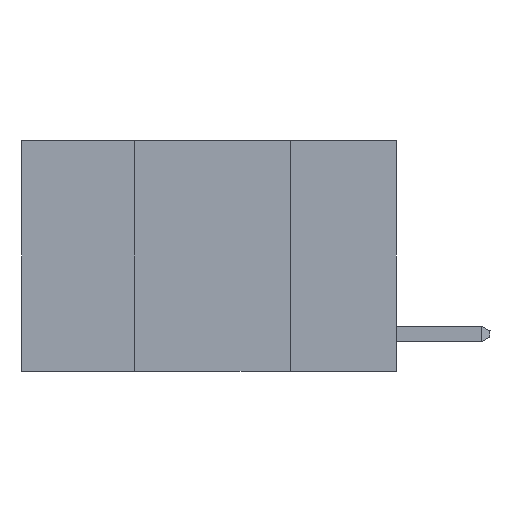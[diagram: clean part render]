
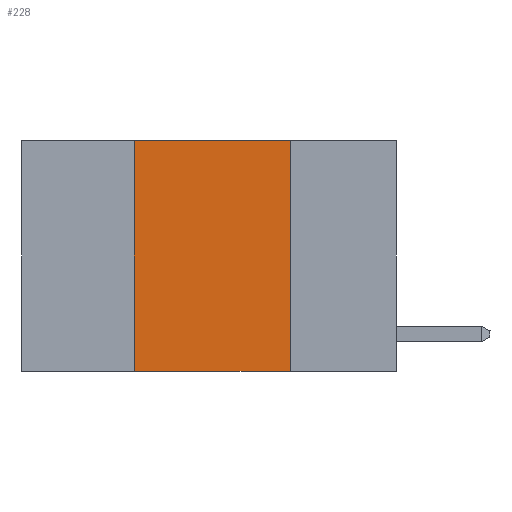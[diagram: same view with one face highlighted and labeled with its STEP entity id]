
A CAD part, left-side view. The second image highlights one B-rep face of the part: STEP entity #228.
In plain terms, the highlighted planar face has unit normal (-1, 0, 0).
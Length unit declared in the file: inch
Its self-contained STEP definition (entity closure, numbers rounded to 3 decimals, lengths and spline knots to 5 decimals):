
#221 = CARTESIAN_POINT ( 'NONE',  ( 0., 0.17, 0. ) ) ;
#228 = ADVANCED_FACE ( 'NONE', ( #13251 ), #10361, .F. ) ;
#314 = LINE ( 'NONE', #221, #16505 ) ;
#476 = DIRECTION ( 'NONE',  ( 0., 0., 1. ) ) ;
#1614 = DIRECTION ( 'NONE',  ( 0., 0., -1. ) ) ;
#2286 = CARTESIAN_POINT ( 'NONE',  ( 0., 0.42, -0.37 ) ) ;
#2450 = VECTOR ( 'NONE', #476, 39.37008 ) ;
#2618 = ORIENTED_EDGE ( 'NONE', *, *, #18844, .F. ) ;
#3694 = VERTEX_POINT ( 'NONE', #2286 ) ;
#4762 = EDGE_LOOP ( 'NONE', ( #12963, #16626, #2618, #14674 ) ) ;
#5062 = VECTOR ( 'NONE', #12794, 39.37008 ) ;
#6056 = LINE ( 'NONE', #15161, #2450 ) ;
#6149 = LINE ( 'NONE', #16313, #10739 ) ;
#6252 = DIRECTION ( 'NONE',  ( 0., -1., 0. ) ) ;
#7243 = EDGE_CURVE ( 'NONE', #9831, #11686, #314, .T. ) ;
#9831 = VERTEX_POINT ( 'NONE', #17787 ) ;
#10361 = PLANE ( 'NONE',  #14960 ) ;
#10739 = VECTOR ( 'NONE', #6252, 39.37008 ) ;
#11539 = CARTESIAN_POINT ( 'NONE',  ( 0., 0.6, 0. ) ) ;
#11686 = VERTEX_POINT ( 'NONE', #13102 ) ;
#12794 = DIRECTION ( 'NONE',  ( 0., -1., 0. ) ) ;
#12963 = ORIENTED_EDGE ( 'NONE', *, *, #7243, .F. ) ;
#12973 = DIRECTION ( 'NONE',  ( 1., 0., 0. ) ) ;
#13102 = CARTESIAN_POINT ( 'NONE',  ( 0., 0.17, -0.37 ) ) ;
#13251 = FACE_OUTER_BOUND ( 'NONE', #4762, .T. ) ;
#13978 = VERTEX_POINT ( 'NONE', #18944 ) ;
#14501 = LINE ( 'NONE', #11539, #5062 ) ;
#14674 = ORIENTED_EDGE ( 'NONE', *, *, #18927, .T. ) ;
#14758 = CARTESIAN_POINT ( 'NONE',  ( 0., 0.6, 0. ) ) ;
#14960 = AXIS2_PLACEMENT_3D ( 'NONE', #14758, #12973, #1614 ) ;
#15161 = CARTESIAN_POINT ( 'NONE',  ( 0., 0.42, 0. ) ) ;
#16313 = CARTESIAN_POINT ( 'NONE',  ( 0., 0.6, -0.37 ) ) ;
#16505 = VECTOR ( 'NONE', #17945, 39.37008 ) ;
#16626 = ORIENTED_EDGE ( 'NONE', *, *, #17363, .F. ) ;
#17363 = EDGE_CURVE ( 'NONE', #13978, #9831, #14501, .T. ) ;
#17787 = CARTESIAN_POINT ( 'NONE',  ( 0., 0.17, 0. ) ) ;
#17945 = DIRECTION ( 'NONE',  ( 0., 0., -1. ) ) ;
#18844 = EDGE_CURVE ( 'NONE', #3694, #13978, #6056, .T. ) ;
#18927 = EDGE_CURVE ( 'NONE', #3694, #11686, #6149, .T. ) ;
#18944 = CARTESIAN_POINT ( 'NONE',  ( 0., 0.42, 0. ) ) ;
